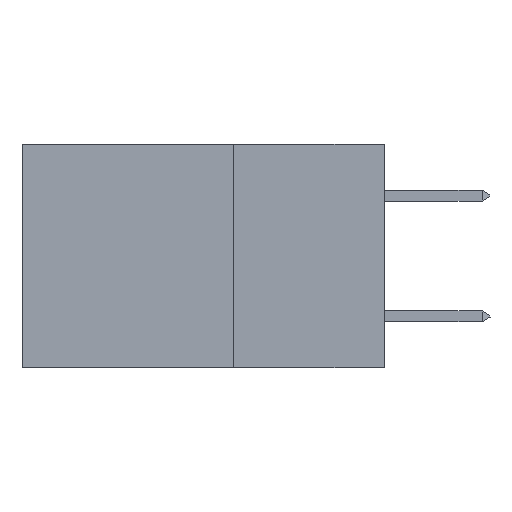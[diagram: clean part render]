
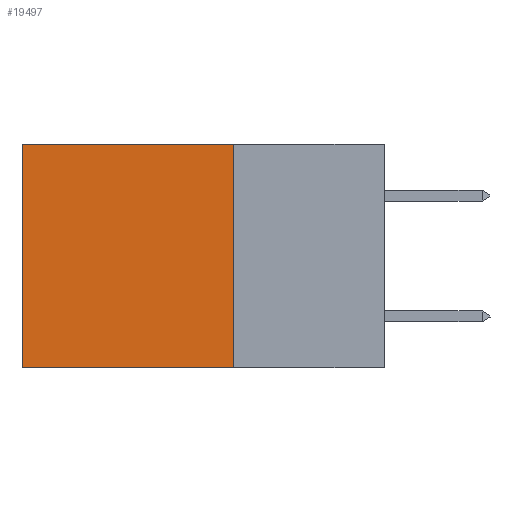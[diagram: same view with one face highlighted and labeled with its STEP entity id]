
A CAD part, left-side view. The second image highlights one B-rep face of the part: STEP entity #19497.
In plain terms, the highlighted planar face has unit normal (-1, 0, 0).
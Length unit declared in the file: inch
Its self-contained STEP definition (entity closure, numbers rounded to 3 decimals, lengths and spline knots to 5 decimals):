
#223 = VERTEX_POINT ( 'NONE', #10732 ) ;
#232 = CARTESIAN_POINT ( 'NONE',  ( 0.2875, 0.6, 0. ) ) ;
#800 = CARTESIAN_POINT ( 'NONE',  ( 0.2875, 0.25, 0. ) ) ;
#1155 = DIRECTION ( 'NONE',  ( 1., 0., 0. ) ) ;
#1360 = CARTESIAN_POINT ( 'NONE',  ( 0.2875, 0.25, 0. ) ) ;
#1404 = ORIENTED_EDGE ( 'NONE', *, *, #11957, .T. ) ;
#1811 = CARTESIAN_POINT ( 'NONE',  ( 0.2875, 0.25, 0. ) ) ;
#2430 = LINE ( 'NONE', #232, #26520 ) ;
#2805 = VECTOR ( 'NONE', #3469, 39.37008 ) ;
#2938 = VECTOR ( 'NONE', #7516, 39.37008 ) ;
#3469 = DIRECTION ( 'NONE',  ( 0., 0., -1. ) ) ;
#4449 = EDGE_CURVE ( 'NONE', #21336, #11668, #2430, .T. ) ;
#5363 = CARTESIAN_POINT ( 'NONE',  ( 0.2875, 0.25, -0.37 ) ) ;
#7404 = CARTESIAN_POINT ( 'NONE',  ( 0.2875, 0.6, 0. ) ) ;
#7516 = DIRECTION ( 'NONE',  ( 0., 1., 0. ) ) ;
#8235 = LINE ( 'NONE', #1360, #2805 ) ;
#8603 = FACE_OUTER_BOUND ( 'NONE', #15632, .T. ) ;
#9096 = ORIENTED_EDGE ( 'NONE', *, *, #4449, .T. ) ;
#10627 = CARTESIAN_POINT ( 'NONE',  ( 0.2875, 0.25, 0. ) ) ;
#10732 = CARTESIAN_POINT ( 'NONE',  ( 0.2875, 0.25, -0.37 ) ) ;
#11668 = VERTEX_POINT ( 'NONE', #23303 ) ;
#11775 = EDGE_CURVE ( 'NONE', #19985, #223, #8235, .T. ) ;
#11957 = EDGE_CURVE ( 'NONE', #19985, #21336, #22997, .T. ) ;
#12076 = VECTOR ( 'NONE', #22104, 39.37008 ) ;
#14795 = LINE ( 'NONE', #5363, #2938 ) ;
#15632 = EDGE_LOOP ( 'NONE', ( #9096, #20756, #25411, #1404 ) ) ;
#19497 = ADVANCED_FACE ( 'NONE', ( #8603 ), #23603, .F. ) ;
#19985 = VERTEX_POINT ( 'NONE', #10627 ) ;
#20756 = ORIENTED_EDGE ( 'NONE', *, *, #25412, .F. ) ;
#21336 = VERTEX_POINT ( 'NONE', #7404 ) ;
#22104 = DIRECTION ( 'NONE',  ( 0., 1., 0. ) ) ;
#22997 = LINE ( 'NONE', #1811, #12076 ) ;
#23303 = CARTESIAN_POINT ( 'NONE',  ( 0.2875, 0.6, -0.37 ) ) ;
#23603 = PLANE ( 'NONE',  #24009 ) ;
#23938 = DIRECTION ( 'NONE',  ( 0., 0., -1. ) ) ;
#24009 = AXIS2_PLACEMENT_3D ( 'NONE', #800, #1155, #25785 ) ;
#25411 = ORIENTED_EDGE ( 'NONE', *, *, #11775, .F. ) ;
#25412 = EDGE_CURVE ( 'NONE', #223, #11668, #14795, .T. ) ;
#25785 = DIRECTION ( 'NONE',  ( 0., 0., -1. ) ) ;
#26520 = VECTOR ( 'NONE', #23938, 39.37008 ) ;
